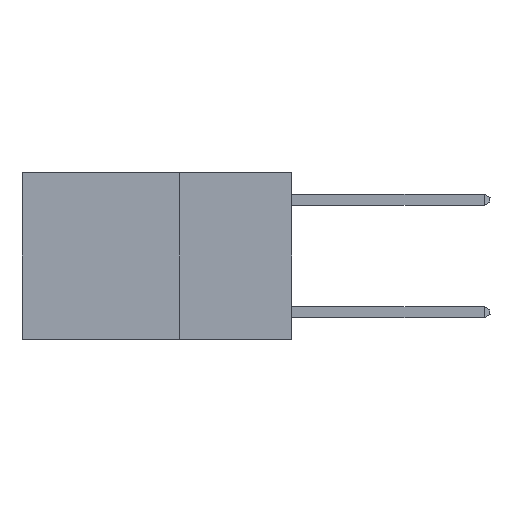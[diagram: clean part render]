
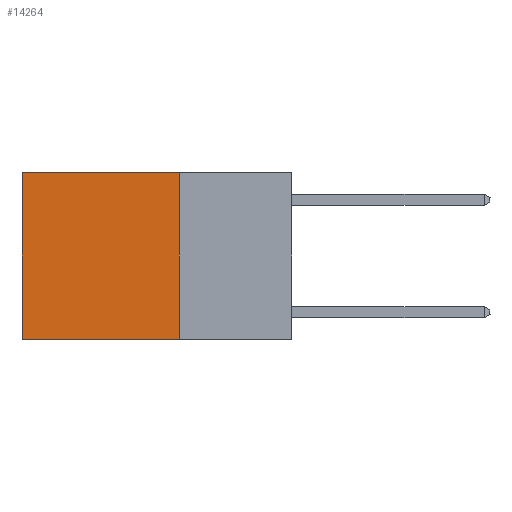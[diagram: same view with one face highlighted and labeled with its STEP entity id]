
A CAD part, left-side view. The second image highlights one B-rep face of the part: STEP entity #14264.
In plain terms, the highlighted planar face has unit normal (-1, 0, 0).
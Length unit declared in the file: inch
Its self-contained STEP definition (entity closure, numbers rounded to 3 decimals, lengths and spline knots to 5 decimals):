
#433 = CARTESIAN_POINT ( 'NONE',  ( 0.2625, 0.25, -0.37 ) ) ;
#782 = VECTOR ( 'NONE', #1405, 39.37008 ) ;
#1089 = PLANE ( 'NONE',  #16386 ) ;
#1105 = ORIENTED_EDGE ( 'NONE', *, *, #6475, .F. ) ;
#1326 = VERTEX_POINT ( 'NONE', #5794 ) ;
#1405 = DIRECTION ( 'NONE',  ( 0., 0., -1. ) ) ;
#2434 = DIRECTION ( 'NONE',  ( 0., 0., -1. ) ) ;
#2594 = LINE ( 'NONE', #11525, #782 ) ;
#3840 = LINE ( 'NONE', #10389, #10330 ) ;
#3915 = FACE_OUTER_BOUND ( 'NONE', #6395, .T. ) ;
#3928 = CARTESIAN_POINT ( 'NONE',  ( 0.2625, 0.25, -0.37 ) ) ;
#4774 = VERTEX_POINT ( 'NONE', #433 ) ;
#5038 = EDGE_CURVE ( 'NONE', #10517, #4774, #3840, .T. ) ;
#5794 = CARTESIAN_POINT ( 'NONE',  ( 0.2625, 0.6, 0. ) ) ;
#6146 = CARTESIAN_POINT ( 'NONE',  ( 0.2625, 0.25, 0. ) ) ;
#6395 = EDGE_LOOP ( 'NONE', ( #11527, #1105, #13795, #12450 ) ) ;
#6475 = EDGE_CURVE ( 'NONE', #4774, #9968, #15323, .T. ) ;
#7969 = DIRECTION ( 'NONE',  ( 0., 1., 0. ) ) ;
#8802 = CARTESIAN_POINT ( 'NONE',  ( 0.2625, 0.6, -0.37 ) ) ;
#9889 = EDGE_CURVE ( 'NONE', #1326, #9968, #2594, .T. ) ;
#9968 = VERTEX_POINT ( 'NONE', #8802 ) ;
#10330 = VECTOR ( 'NONE', #12740, 39.37008 ) ;
#10389 = CARTESIAN_POINT ( 'NONE',  ( 0.2625, 0.25, 0. ) ) ;
#10517 = VERTEX_POINT ( 'NONE', #11834 ) ;
#11199 = DIRECTION ( 'NONE',  ( 1., 0., 0. ) ) ;
#11525 = CARTESIAN_POINT ( 'NONE',  ( 0.2625, 0.6, 0. ) ) ;
#11527 = ORIENTED_EDGE ( 'NONE', *, *, #9889, .T. ) ;
#11622 = LINE ( 'NONE', #15648, #12635 ) ;
#11834 = CARTESIAN_POINT ( 'NONE',  ( 0.2625, 0.25, 0. ) ) ;
#12450 = ORIENTED_EDGE ( 'NONE', *, *, #14300, .T. ) ;
#12635 = VECTOR ( 'NONE', #7969, 39.37008 ) ;
#12740 = DIRECTION ( 'NONE',  ( 0., 0., -1. ) ) ;
#13795 = ORIENTED_EDGE ( 'NONE', *, *, #5038, .F. ) ;
#14083 = DIRECTION ( 'NONE',  ( 0., 1., 0. ) ) ;
#14264 = ADVANCED_FACE ( 'NONE', ( #3915 ), #1089, .F. ) ;
#14300 = EDGE_CURVE ( 'NONE', #10517, #1326, #11622, .T. ) ;
#15323 = LINE ( 'NONE', #3928, #15456 ) ;
#15456 = VECTOR ( 'NONE', #14083, 39.37008 ) ;
#15648 = CARTESIAN_POINT ( 'NONE',  ( 0.2625, 0.25, 0. ) ) ;
#16386 = AXIS2_PLACEMENT_3D ( 'NONE', #6146, #11199, #2434 ) ;
